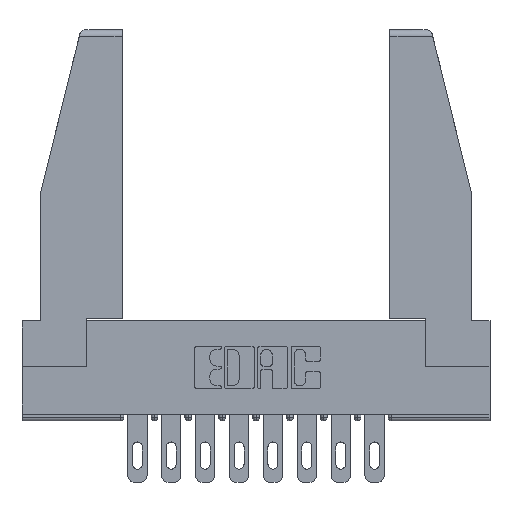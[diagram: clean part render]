
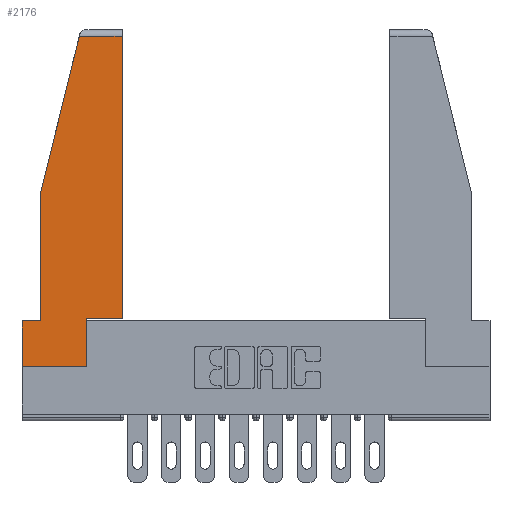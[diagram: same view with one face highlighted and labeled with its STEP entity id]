
A CAD part, top view. The second image highlights one B-rep face of the part: STEP entity #2176.
In plain terms, the highlighted planar face has unit normal (0, 0, 1).
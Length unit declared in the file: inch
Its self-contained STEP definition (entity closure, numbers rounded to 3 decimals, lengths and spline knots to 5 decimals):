
#124 = VERTEX_POINT ( 'NONE', #6831 ) ;
#256 = VECTOR ( 'NONE', #12518, 39.37008 ) ;
#420 = LINE ( 'NONE', #2099, #5222 ) ;
#1094 = CARTESIAN_POINT ( 'NONE',  ( 0.461, 0.223, 0. ) ) ;
#1108 = PLANE ( 'NONE',  #14186 ) ;
#1169 = DIRECTION ( 'NONE',  ( 0., 0., 1. ) ) ;
#1602 = EDGE_CURVE ( 'NONE', #14120, #13741, #3792, .T. ) ;
#1914 = DIRECTION ( 'NONE',  ( 0., -1., 0. ) ) ;
#2025 = EDGE_CURVE ( 'NONE', #124, #14975, #12417, .T. ) ;
#2099 = CARTESIAN_POINT ( 'NONE',  ( 0.271, 1.55, 0. ) ) ;
#2176 = ADVANCED_FACE ( 'NONE', ( #6709 ), #1108, .T. ) ;
#2656 = VERTEX_POINT ( 'NONE', #11776 ) ;
#2691 = LINE ( 'NONE', #3198, #5447 ) ;
#2692 = EDGE_CURVE ( 'NONE', #10217, #2656, #420, .T. ) ;
#2738 = DIRECTION ( 'NONE',  ( 0., 1., 0. ) ) ;
#2925 = CARTESIAN_POINT ( 'NONE',  ( 0., 0.21, 0. ) ) ;
#3198 = CARTESIAN_POINT ( 'NONE',  ( 0.086, 0.8, 0. ) ) ;
#3338 = ORIENTED_EDGE ( 'NONE', *, *, #2692, .T. ) ;
#3474 = ORIENTED_EDGE ( 'NONE', *, *, #13340, .T. ) ;
#3745 = CARTESIAN_POINT ( 'NONE',  ( 0.297, 0., 0. ) ) ;
#3792 = LINE ( 'NONE', #6560, #256 ) ;
#3925 = LINE ( 'NONE', #7587, #7058 ) ;
#3983 = DIRECTION ( 'NONE',  ( 0., -1., 0. ) ) ;
#4026 = CARTESIAN_POINT ( 'NONE',  ( 0.2636, 1.52, 0. ) ) ;
#4362 = DIRECTION ( 'NONE',  ( -1., 0., 0. ) ) ;
#4732 = EDGE_CURVE ( 'NONE', #12413, #10217, #3925, .T. ) ;
#5222 = VECTOR ( 'NONE', #15287, 39.37008 ) ;
#5334 = VECTOR ( 'NONE', #9348, 39.37008 ) ;
#5447 = VECTOR ( 'NONE', #1914, 39.37008 ) ;
#5549 = VERTEX_POINT ( 'NONE', #6430 ) ;
#5573 = VERTEX_POINT ( 'NONE', #9919 ) ;
#5683 = ORIENTED_EDGE ( 'NONE', *, *, #2025, .T. ) ;
#5818 = DIRECTION ( 'NONE',  ( 1., 0., 0. ) ) ;
#5843 = CARTESIAN_POINT ( 'NONE',  ( 0., 0., 0. ) ) ;
#5897 = EDGE_LOOP ( 'NONE', ( #7675, #5962, #3338, #3474, #5683, #7987, #6475, #8561, #10844 ) ) ;
#5916 = CARTESIAN_POINT ( 'NONE',  ( 0., 0., 0. ) ) ;
#5962 = ORIENTED_EDGE ( 'NONE', *, *, #4732, .T. ) ;
#6145 = VECTOR ( 'NONE', #4362, 39.37008 ) ;
#6422 = DIRECTION ( 'NONE',  ( -1., 0., 0. ) ) ;
#6430 = CARTESIAN_POINT ( 'NONE',  ( 0., 0., 0. ) ) ;
#6431 = VECTOR ( 'NONE', #5818, 39.37008 ) ;
#6475 = ORIENTED_EDGE ( 'NONE', *, *, #12115, .T. ) ;
#6560 = CARTESIAN_POINT ( 'NONE',  ( 0.297, 0.223, 0. ) ) ;
#6709 = FACE_OUTER_BOUND ( 'NONE', #5897, .T. ) ;
#6831 = CARTESIAN_POINT ( 'NONE',  ( 0.086, 0.21, 0. ) ) ;
#7058 = VECTOR ( 'NONE', #6422, 39.37008 ) ;
#7189 = LINE ( 'NONE', #1094, #5334 ) ;
#7587 = CARTESIAN_POINT ( 'NONE',  ( 0., 1.52, 0. ) ) ;
#7675 = ORIENTED_EDGE ( 'NONE', *, *, #11659, .T. ) ;
#7939 = CARTESIAN_POINT ( 'NONE',  ( 0., 0.21, 0. ) ) ;
#7987 = ORIENTED_EDGE ( 'NONE', *, *, #12879, .T. ) ;
#8561 = ORIENTED_EDGE ( 'NONE', *, *, #13487, .T. ) ;
#8767 = CARTESIAN_POINT ( 'NONE',  ( 0.461, 1.52, 0. ) ) ;
#9348 = DIRECTION ( 'NONE',  ( 0., 1., 0. ) ) ;
#9705 = LINE ( 'NONE', #3745, #12462 ) ;
#9919 = CARTESIAN_POINT ( 'NONE',  ( 0.297, 0., 0. ) ) ;
#9920 = LINE ( 'NONE', #5916, #6431 ) ;
#10217 = VERTEX_POINT ( 'NONE', #4026 ) ;
#10844 = ORIENTED_EDGE ( 'NONE', *, *, #1602, .T. ) ;
#10994 = LINE ( 'NONE', #2925, #15247 ) ;
#11659 = EDGE_CURVE ( 'NONE', #13741, #12413, #7189, .T. ) ;
#11776 = CARTESIAN_POINT ( 'NONE',  ( 0.086, 0.8, 0. ) ) ;
#11872 = DIRECTION ( 'NONE',  ( 1., 0., 0. ) ) ;
#12115 = EDGE_CURVE ( 'NONE', #5549, #5573, #9920, .T. ) ;
#12413 = VERTEX_POINT ( 'NONE', #8767 ) ;
#12417 = LINE ( 'NONE', #7939, #6145 ) ;
#12462 = VECTOR ( 'NONE', #2738, 39.37008 ) ;
#12518 = DIRECTION ( 'NONE',  ( 1., 0., 0. ) ) ;
#12879 = EDGE_CURVE ( 'NONE', #14975, #5549, #10994, .T. ) ;
#13094 = CARTESIAN_POINT ( 'NONE',  ( 0.297, 0.223, 0. ) ) ;
#13340 = EDGE_CURVE ( 'NONE', #2656, #124, #2691, .T. ) ;
#13487 = EDGE_CURVE ( 'NONE', #5573, #14120, #9705, .T. ) ;
#13741 = VERTEX_POINT ( 'NONE', #14787 ) ;
#14120 = VERTEX_POINT ( 'NONE', #13094 ) ;
#14186 = AXIS2_PLACEMENT_3D ( 'NONE', #5843, #1169, #11872 ) ;
#14491 = CARTESIAN_POINT ( 'NONE',  ( 0., 0.21, 0. ) ) ;
#14787 = CARTESIAN_POINT ( 'NONE',  ( 0.461, 0.223, 0. ) ) ;
#14975 = VERTEX_POINT ( 'NONE', #14491 ) ;
#15247 = VECTOR ( 'NONE', #3983, 39.37008 ) ;
#15287 = DIRECTION ( 'NONE',  ( -0.239, -0.971, 0. ) ) ;
